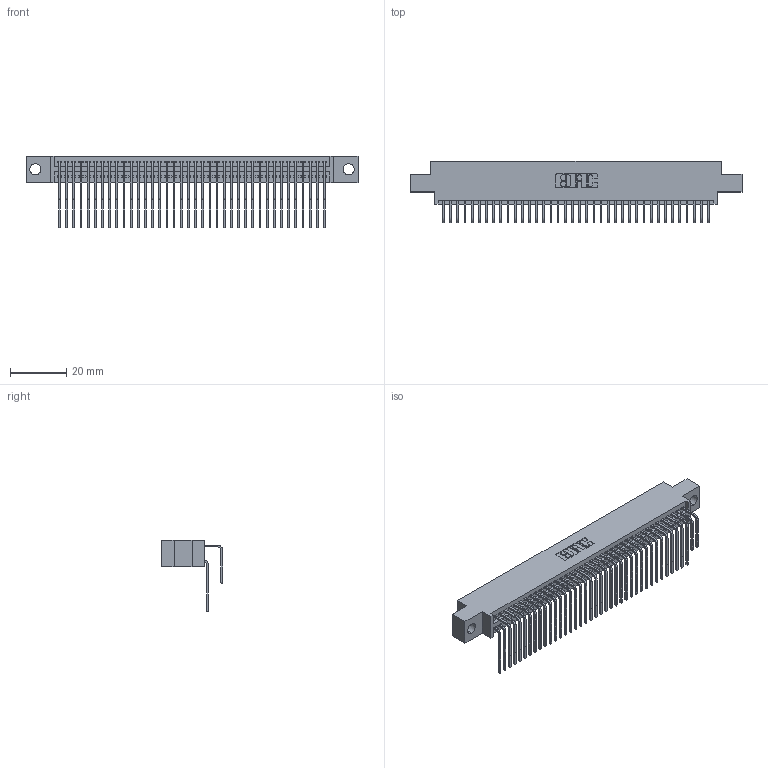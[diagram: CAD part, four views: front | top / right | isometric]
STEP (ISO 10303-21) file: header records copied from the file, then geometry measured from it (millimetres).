
FILE_DESCRIPTION (( 'STEP AP203' ), '1' );
FILE_NAME ('395-076-558-804.STEP', '2018-11-27T22:44:16', ( '' ), ( '' ), 'SwSTEP 2.0', 'SolidWorks 2016', '' );
FILE_SCHEMA (( 'CONFIG_CONTROL_DESIGN' ));
Length unit declared in the file: inch
Products named in the file (4): 345 Part_0.170 Offset - 0.156 Dia-TH; 345-292-001_558 559 Tail - 1; 345-292-001_558 Tail - 2; 395-076-558-804
Assembly tree (77 placements, depth 2):
  395-076-558-804
    345 Part_0.170 Offset - 0.156 Dia-TH
    345-292-001_558 559 Tail - 1  x38
    345-292-001_558 Tail - 2  x38
Bounding box: 117.73 x 21.83 x 25.53 mm (x, y, z)
Volume: 11636.4 mm3; surface area: 19143.3 mm2
Topology: 77 solids, 77 shells, 4082 faces, 12133 edges, 7986 vertices
Faces by surface type: plane 2744, cylinder 1338
Entity records: 32141 total; most frequent: CARTESIAN_POINT 5439, ORIENTED_EDGE 5322, DIRECTION 4773, EDGE_CURVE 2661, VECTOR 2337, LINE 2337, VERTEX_POINT 1770, AXIS2_PLACEMENT_3D 1218
